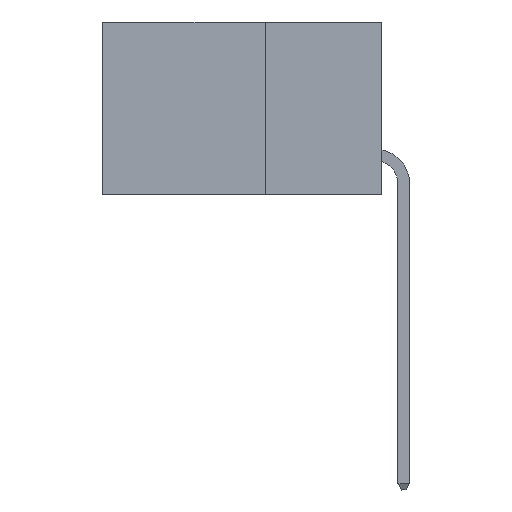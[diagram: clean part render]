
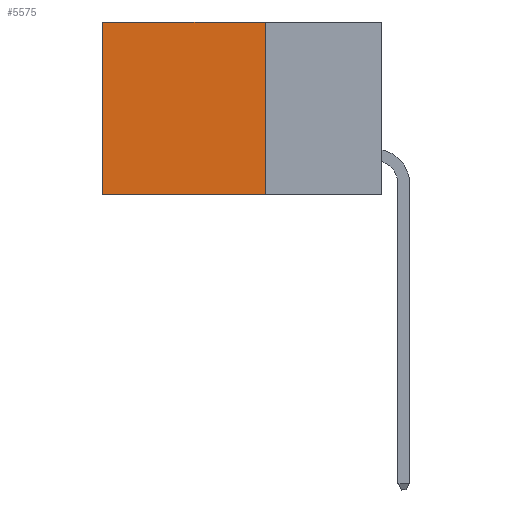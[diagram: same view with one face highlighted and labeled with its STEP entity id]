
A CAD part, left-side view. The second image highlights one B-rep face of the part: STEP entity #5575.
In plain terms, the highlighted planar face has unit normal (-1, 0, 0).
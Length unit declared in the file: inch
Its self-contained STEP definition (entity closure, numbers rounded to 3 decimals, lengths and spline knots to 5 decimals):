
#651 = LINE ( 'NONE', #6564, #14361 ) ;
#1115 = VECTOR ( 'NONE', #1608, 39.37008 ) ;
#1608 = DIRECTION ( 'NONE',  ( 0., 0., -1. ) ) ;
#1758 = FACE_OUTER_BOUND ( 'NONE', #9879, .T. ) ;
#2302 = ORIENTED_EDGE ( 'NONE', *, *, #8048, .F. ) ;
#3095 = DIRECTION ( 'NONE',  ( 1., 0., 0. ) ) ;
#3572 = EDGE_CURVE ( 'NONE', #6976, #12063, #7212, .T. ) ;
#3628 = VECTOR ( 'NONE', #4794, 39.37008 ) ;
#4794 = DIRECTION ( 'NONE',  ( 0., 1., 0. ) ) ;
#5452 = CARTESIAN_POINT ( 'NONE',  ( 0.2875, 0.6, -0.37 ) ) ;
#5575 = ADVANCED_FACE ( 'NONE', ( #1758 ), #13095, .F. ) ;
#6212 = LINE ( 'NONE', #15787, #3628 ) ;
#6564 = CARTESIAN_POINT ( 'NONE',  ( 0.2875, 0.6, 0. ) ) ;
#6976 = VERTEX_POINT ( 'NONE', #9633 ) ;
#6994 = DIRECTION ( 'NONE',  ( 0., 0., -1. ) ) ;
#7212 = LINE ( 'NONE', #12854, #1115 ) ;
#7396 = VERTEX_POINT ( 'NONE', #5452 ) ;
#7728 = DIRECTION ( 'NONE',  ( 0., 1., 0. ) ) ;
#7834 = DIRECTION ( 'NONE',  ( 0., 0., -1. ) ) ;
#8048 = EDGE_CURVE ( 'NONE', #12063, #7396, #6212, .T. ) ;
#9446 = CARTESIAN_POINT ( 'NONE',  ( 0.2875, 0.25, 0. ) ) ;
#9633 = CARTESIAN_POINT ( 'NONE',  ( 0.2875, 0.25, 0. ) ) ;
#9879 = EDGE_LOOP ( 'NONE', ( #15170, #2302, #13654, #15141 ) ) ;
#10530 = VECTOR ( 'NONE', #7728, 39.37008 ) ;
#10867 = EDGE_CURVE ( 'NONE', #6976, #14696, #13816, .T. ) ;
#12063 = VERTEX_POINT ( 'NONE', #15985 ) ;
#12854 = CARTESIAN_POINT ( 'NONE',  ( 0.2875, 0.25, 0. ) ) ;
#13095 = PLANE ( 'NONE',  #13903 ) ;
#13497 = CARTESIAN_POINT ( 'NONE',  ( 0.2875, 0.6, 0. ) ) ;
#13654 = ORIENTED_EDGE ( 'NONE', *, *, #3572, .F. ) ;
#13816 = LINE ( 'NONE', #15320, #10530 ) ;
#13903 = AXIS2_PLACEMENT_3D ( 'NONE', #9446, #3095, #6994 ) ;
#14199 = EDGE_CURVE ( 'NONE', #14696, #7396, #651, .T. ) ;
#14361 = VECTOR ( 'NONE', #7834, 39.37008 ) ;
#14696 = VERTEX_POINT ( 'NONE', #13497 ) ;
#15141 = ORIENTED_EDGE ( 'NONE', *, *, #10867, .T. ) ;
#15170 = ORIENTED_EDGE ( 'NONE', *, *, #14199, .T. ) ;
#15320 = CARTESIAN_POINT ( 'NONE',  ( 0.2875, 0.25, 0. ) ) ;
#15787 = CARTESIAN_POINT ( 'NONE',  ( 0.2875, 0.25, -0.37 ) ) ;
#15985 = CARTESIAN_POINT ( 'NONE',  ( 0.2875, 0.25, -0.37 ) ) ;
